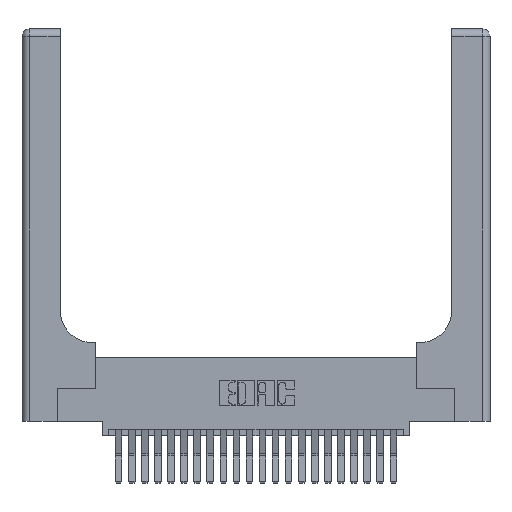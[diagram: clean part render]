
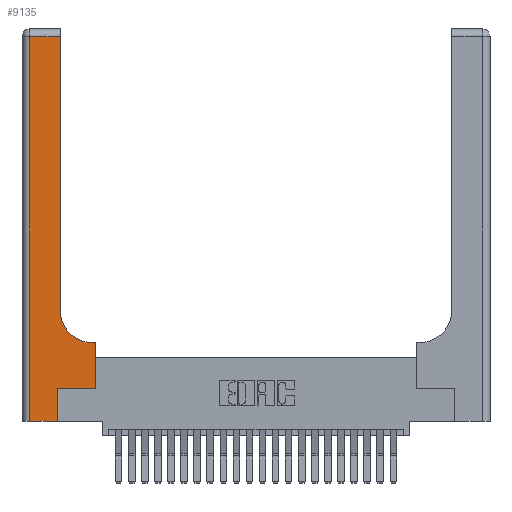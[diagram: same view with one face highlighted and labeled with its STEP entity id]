
A CAD part, top view. The second image highlights one B-rep face of the part: STEP entity #9135.
In plain terms, the highlighted planar face has unit normal (0, 0, 1).
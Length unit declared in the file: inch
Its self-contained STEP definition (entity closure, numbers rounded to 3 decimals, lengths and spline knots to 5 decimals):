
#64 = VERTEX_POINT ( 'NONE', #23305 ) ;
#295 = DIRECTION ( 'NONE',  ( -1., 0., 0. ) ) ;
#366 = ORIENTED_EDGE ( 'NONE', *, *, #24310, .T. ) ;
#370 = VERTEX_POINT ( 'NONE', #16389 ) ;
#626 = CARTESIAN_POINT ( 'NONE',  ( 0.5415, 0.85, 0.37 ) ) ;
#699 = ORIENTED_EDGE ( 'NONE', *, *, #13016, .T. ) ;
#788 = CARTESIAN_POINT ( 'NONE',  ( 0.06, 2.94, 0.37 ) ) ;
#820 = VECTOR ( 'NONE', #11217, 39.37008 ) ;
#1894 = VERTEX_POINT ( 'NONE', #788 ) ;
#1970 = CARTESIAN_POINT ( 'NONE',  ( 0.5585, 0.25, 0.37 ) ) ;
#2661 = DIRECTION ( 'NONE',  ( 1., 0., 0. ) ) ;
#2855 = ORIENTED_EDGE ( 'NONE', *, *, #8312, .T. ) ;
#3395 = VECTOR ( 'NONE', #25288, 39.37008 ) ;
#4020 = LINE ( 'NONE', #7867, #3395 ) ;
#4249 = VERTEX_POINT ( 'NONE', #22763 ) ;
#4606 = DIRECTION ( 'NONE',  ( 0., -1., 0. ) ) ;
#4737 = EDGE_CURVE ( 'NONE', #21798, #21858, #14883, .T. ) ;
#4917 = CARTESIAN_POINT ( 'NONE',  ( 0.269, 0.25, 0.37 ) ) ;
#5145 = ORIENTED_EDGE ( 'NONE', *, *, #13972, .T. ) ;
#5791 = LINE ( 'NONE', #1970, #10485 ) ;
#5831 = EDGE_CURVE ( 'NONE', #1894, #4249, #16369, .T. ) ;
#5868 = VECTOR ( 'NONE', #4606, 39.37008 ) ;
#7294 = EDGE_CURVE ( 'NONE', #23607, #64, #5791, .T. ) ;
#7389 = ORIENTED_EDGE ( 'NONE', *, *, #7294, .T. ) ;
#7867 = CARTESIAN_POINT ( 'NONE',  ( 0.2915, 0.6, 0.37 ) ) ;
#8312 = EDGE_CURVE ( 'NONE', #18456, #1894, #15978, .T. ) ;
#8837 = CARTESIAN_POINT ( 'NONE',  ( 0.2915, 3., 0.37 ) ) ;
#9135 = ADVANCED_FACE ( 'NONE', ( #15008 ), #21887, .F. ) ;
#9360 = EDGE_CURVE ( 'NONE', #19983, #18456, #20539, .T. ) ;
#9668 = VECTOR ( 'NONE', #18988, 39.37008 ) ;
#9928 = LINE ( 'NONE', #11535, #19712 ) ;
#10248 = CARTESIAN_POINT ( 'NONE',  ( 0., 3., 0.37 ) ) ;
#10485 = VECTOR ( 'NONE', #17749, 39.37008 ) ;
#10494 = CARTESIAN_POINT ( 'NONE',  ( 0.06, 3., 0.37 ) ) ;
#10728 = CARTESIAN_POINT ( 'NONE',  ( 0.269, 0., 0.37 ) ) ;
#11217 = DIRECTION ( 'NONE',  ( -1., 0., 0. ) ) ;
#11535 = CARTESIAN_POINT ( 'NONE',  ( 0.269, 0.25, 0.37 ) ) ;
#12221 = DIRECTION ( 'NONE',  ( 0., 0., -1. ) ) ;
#12750 = CARTESIAN_POINT ( 'NONE',  ( 0., 0., 0.37 ) ) ;
#12765 = ORIENTED_EDGE ( 'NONE', *, *, #16560, .T. ) ;
#12881 = EDGE_LOOP ( 'NONE', ( #16902, #2855, #24160, #366, #21530, #12765, #7389, #5145, #699 ) ) ;
#13016 = EDGE_CURVE ( 'NONE', #370, #19983, #21527, .T. ) ;
#13347 = LINE ( 'NONE', #12750, #23051 ) ;
#13972 = EDGE_CURVE ( 'NONE', #64, #370, #4020, .T. ) ;
#14488 = DIRECTION ( 'NONE',  ( 0., 0., -1. ) ) ;
#14702 = DIRECTION ( 'NONE',  ( 1., 0., 0. ) ) ;
#14883 = LINE ( 'NONE', #17004, #9668 ) ;
#15008 = FACE_OUTER_BOUND ( 'NONE', #12881, .T. ) ;
#15341 = VECTOR ( 'NONE', #20642, 39.37008 ) ;
#15364 = CARTESIAN_POINT ( 'NONE',  ( 0.2915, 0.85, 0.37 ) ) ;
#15446 = CARTESIAN_POINT ( 'NONE',  ( 0.2915, 2.94, 0.37 ) ) ;
#15978 = LINE ( 'NONE', #20916, #820 ) ;
#16068 = AXIS2_PLACEMENT_3D ( 'NONE', #626, #14488, #2661 ) ;
#16369 = LINE ( 'NONE', #10494, #5868 ) ;
#16389 = CARTESIAN_POINT ( 'NONE',  ( 0.5415, 0.6, 0.37 ) ) ;
#16560 = EDGE_CURVE ( 'NONE', #21858, #23607, #9928, .T. ) ;
#16902 = ORIENTED_EDGE ( 'NONE', *, *, #9360, .T. ) ;
#17004 = CARTESIAN_POINT ( 'NONE',  ( 0.269, 0., 0.37 ) ) ;
#17749 = DIRECTION ( 'NONE',  ( 0., 1., 0. ) ) ;
#18456 = VERTEX_POINT ( 'NONE', #15446 ) ;
#18800 = AXIS2_PLACEMENT_3D ( 'NONE', #10248, #12221, #295 ) ;
#18988 = DIRECTION ( 'NONE',  ( 0., 1., 0. ) ) ;
#19275 = DIRECTION ( 'NONE',  ( 1., 0., 0. ) ) ;
#19712 = VECTOR ( 'NONE', #19275, 39.37008 ) ;
#19983 = VERTEX_POINT ( 'NONE', #15364 ) ;
#20539 = LINE ( 'NONE', #8837, #15341 ) ;
#20642 = DIRECTION ( 'NONE',  ( 0., 1., 0. ) ) ;
#20916 = CARTESIAN_POINT ( 'NONE',  ( 0., 2.94, 0.37 ) ) ;
#21527 = CIRCLE ( 'NONE', #16068, 0.25 ) ;
#21530 = ORIENTED_EDGE ( 'NONE', *, *, #4737, .T. ) ;
#21771 = CARTESIAN_POINT ( 'NONE',  ( 0.5585, 0.25, 0.37 ) ) ;
#21798 = VERTEX_POINT ( 'NONE', #10728 ) ;
#21858 = VERTEX_POINT ( 'NONE', #4917 ) ;
#21887 = PLANE ( 'NONE',  #18800 ) ;
#22763 = CARTESIAN_POINT ( 'NONE',  ( 0.06, 0., 0.37 ) ) ;
#23051 = VECTOR ( 'NONE', #14702, 39.37008 ) ;
#23305 = CARTESIAN_POINT ( 'NONE',  ( 0.5585, 0.6, 0.37 ) ) ;
#23607 = VERTEX_POINT ( 'NONE', #21771 ) ;
#24160 = ORIENTED_EDGE ( 'NONE', *, *, #5831, .T. ) ;
#24310 = EDGE_CURVE ( 'NONE', #4249, #21798, #13347, .T. ) ;
#25288 = DIRECTION ( 'NONE',  ( -1., 0., 0. ) ) ;
